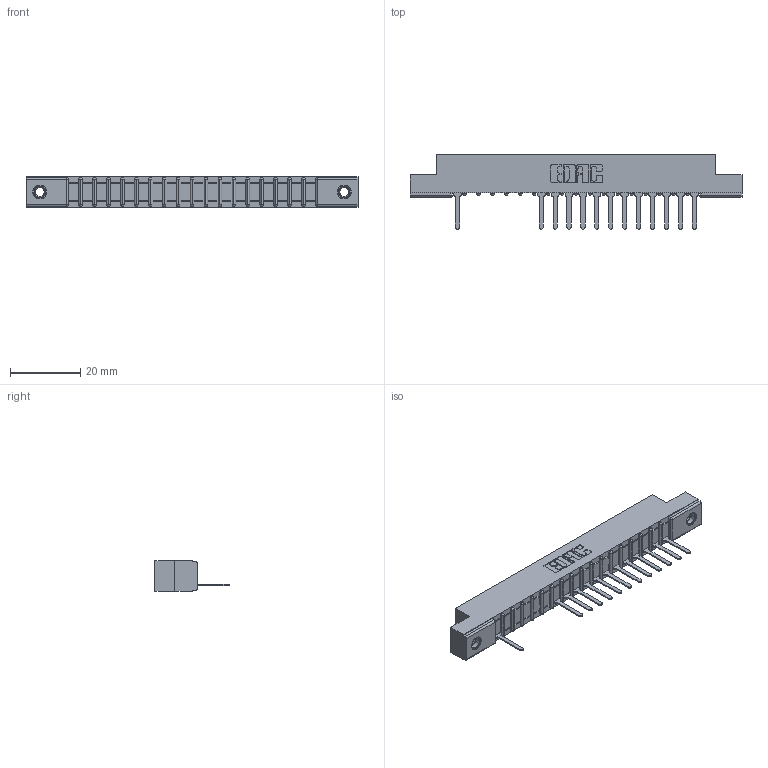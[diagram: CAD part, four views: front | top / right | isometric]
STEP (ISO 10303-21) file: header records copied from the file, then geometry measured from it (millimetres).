
FILE_DESCRIPTION (( 'STEP AP203' ), '1' );
FILE_NAME ('357-018-527-107.STEP', '2018-08-08T04:24:52', ( '' ), ( '' ), 'SwSTEP 2.0', 'SolidWorks 2016', '' );
FILE_SCHEMA (( 'CONFIG_CONTROL_DESIGN' ));
Length unit declared in the file: inch
Products named in the file (4): 307-290-001_527; 345-250-001_345-250-005-103; 357-018-527-107; 307 Part_.156 Dia Mounting Holes
Assembly tree (16 placements, depth 2):
  357-018-527-107
    307 Part_.156 Dia Mounting Holes
    307-290-001_527  x13
    345-250-001_345-250-005-103  x2
Bounding box: 94.34 x 21.11 x 8.71 mm (x, y, z)
Volume: 5888.3 mm3; surface area: 8621.5 mm2
Topology: 16 solids, 16 shells, 1025 faces, 2885 edges, 1846 vertices
Faces by surface type: plane 643, cylinder 328, sphere 38, cone 12, torus 4
Entity records: 19383 total; most frequent: CARTESIAN_POINT 3258, ORIENTED_EDGE 3242, DIRECTION 3187, EDGE_CURVE 1621, LINE 1233, VECTOR 1233, VERTEX_POINT 1048, AXIS2_PLACEMENT_3D 977
